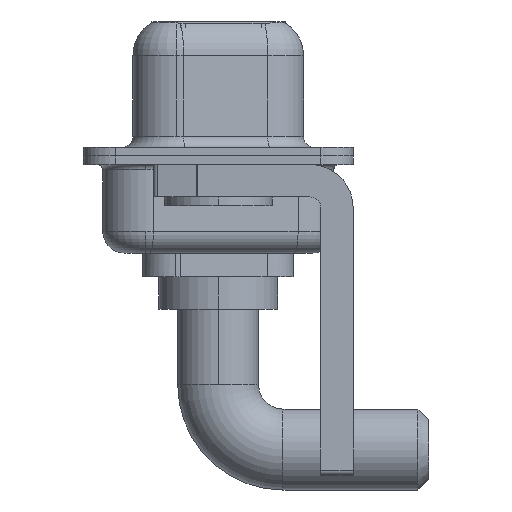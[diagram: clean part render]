
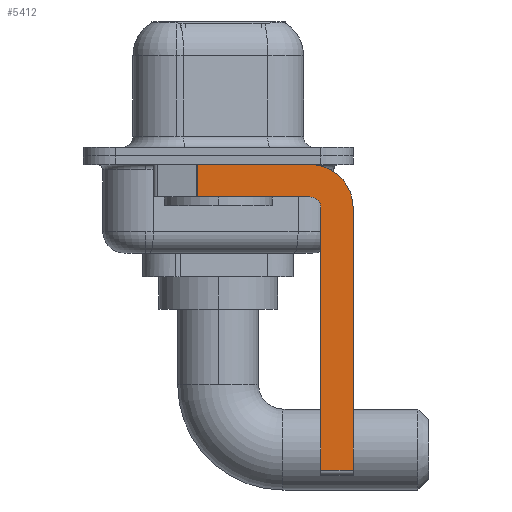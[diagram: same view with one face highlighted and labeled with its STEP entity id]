
A CAD part, left-side view. The second image highlights one B-rep face of the part: STEP entity #5412.
In plain terms, the highlighted planar face has unit normal (-1, 0, 0).
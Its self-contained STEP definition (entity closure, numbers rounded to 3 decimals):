
#215 = VERTEX_POINT ( 'NONE', #4881 ) ;
#233 = DIRECTION ( 'NONE',  ( 0., 0., 1. ) ) ;
#318 = ORIENTED_EDGE ( 'NONE', *, *, #12739, .F. ) ;
#354 = AXIS2_PLACEMENT_3D ( 'NONE', #10210, #6829, #233 ) ;
#401 = VERTEX_POINT ( 'NONE', #9408 ) ;
#510 = EDGE_CURVE ( 'NONE', #3504, #9815, #6223, .T. ) ;
#586 = LINE ( 'NONE', #10084, #4922 ) ;
#731 = VERTEX_POINT ( 'NONE', #3389 ) ;
#924 = VECTOR ( 'NONE', #4280, 1000. ) ;
#963 = VERTEX_POINT ( 'NONE', #9392 ) ;
#1815 = ORIENTED_EDGE ( 'NONE', *, *, #3569, .F. ) ;
#1819 = DIRECTION ( 'NONE',  ( 1., 0., 0. ) ) ;
#1864 = LINE ( 'NONE', #13706, #4674 ) ;
#2394 = VERTEX_POINT ( 'NONE', #5501 ) ;
#2588 = CARTESIAN_POINT ( 'NONE',  ( -2.9, 0.978, -0.4 ) ) ;
#3221 = EDGE_CURVE ( 'NONE', #3504, #401, #6413, .T. ) ;
#3389 = CARTESIAN_POINT ( 'NONE',  ( -2.9, -4.75, -2.4 ) ) ;
#3504 = VERTEX_POINT ( 'NONE', #2588 ) ;
#3560 = VECTOR ( 'NONE', #4054, 1000. ) ;
#3569 = EDGE_CURVE ( 'NONE', #215, #731, #9084, .T. ) ;
#3638 = DIRECTION ( 'NONE',  ( 0., 0., 1. ) ) ;
#4054 = DIRECTION ( 'NONE',  ( 0., 0., -1. ) ) ;
#4280 = DIRECTION ( 'NONE',  ( 0., -1., 0. ) ) ;
#4385 = ORIENTED_EDGE ( 'NONE', *, *, #10401, .T. ) ;
#4420 = VECTOR ( 'NONE', #8425, 1000. ) ;
#4551 = DIRECTION ( 'NONE',  ( 0., 0., -1. ) ) ;
#4674 = VECTOR ( 'NONE', #13566, 1000. ) ;
#4881 = CARTESIAN_POINT ( 'NONE',  ( -2.9, -4.75, -14.55 ) ) ;
#4912 = CARTESIAN_POINT ( 'NONE',  ( -2.9, 0.978, -1.9 ) ) ;
#4917 = DIRECTION ( 'NONE',  ( 0., 1., 0. ) ) ;
#4922 = VECTOR ( 'NONE', #4917, 1000. ) ;
#4967 = ORIENTED_EDGE ( 'NONE', *, *, #3221, .F. ) ;
#4977 = CARTESIAN_POINT ( 'NONE',  ( -2.9, -4.75, -14.8 ) ) ;
#5160 = CARTESIAN_POINT ( 'NONE',  ( -2.9, 0.978, -1.9 ) ) ;
#5412 = ADVANCED_FACE ( 'NONE', ( #12219 ), #8739, .F. ) ;
#5501 = CARTESIAN_POINT ( 'NONE',  ( -2.9, -4.25, -1.9 ) ) ;
#5654 = ORIENTED_EDGE ( 'NONE', *, *, #9717, .F. ) ;
#6118 = CARTESIAN_POINT ( 'NONE',  ( -2.9, -4.25, -2.4 ) ) ;
#6223 = LINE ( 'NONE', #5160, #4420 ) ;
#6413 = LINE ( 'NONE', #8612, #924 ) ;
#6829 = DIRECTION ( 'NONE',  ( -1., 0., 0. ) ) ;
#7475 = ORIENTED_EDGE ( 'NONE', *, *, #13992, .F. ) ;
#7681 = DIRECTION ( 'NONE',  ( 1., 0., 0. ) ) ;
#8119 = DIRECTION ( 'NONE',  ( 0., 0., -1. ) ) ;
#8425 = DIRECTION ( 'NONE',  ( 0., 0., -1. ) ) ;
#8444 = LINE ( 'NONE', #12781, #3560 ) ;
#8612 = CARTESIAN_POINT ( 'NONE',  ( -2.9, 3., -0.4 ) ) ;
#8739 = PLANE ( 'NONE',  #9556 ) ;
#8808 = CARTESIAN_POINT ( 'NONE',  ( -2.9, -4.25, -2.4 ) ) ;
#9084 = LINE ( 'NONE', #4977, #13875 ) ;
#9392 = CARTESIAN_POINT ( 'NONE',  ( -2.9, -6.25, -2.4 ) ) ;
#9408 = CARTESIAN_POINT ( 'NONE',  ( -2.9, -4.25, -0.4 ) ) ;
#9468 = CIRCLE ( 'NONE', #11288, 2. ) ;
#9556 = AXIS2_PLACEMENT_3D ( 'NONE', #8808, #7681, #4551 ) ;
#9717 = EDGE_CURVE ( 'NONE', #731, #2394, #10082, .T. ) ;
#9815 = VERTEX_POINT ( 'NONE', #4912 ) ;
#10082 = CIRCLE ( 'NONE', #354, 0.5 ) ;
#10084 = CARTESIAN_POINT ( 'NONE',  ( -2.9, -4.25, -1.9 ) ) ;
#10210 = CARTESIAN_POINT ( 'NONE',  ( -2.9, -4.25, -2.4 ) ) ;
#10401 = EDGE_CURVE ( 'NONE', #215, #11732, #1864, .T. ) ;
#10906 = ORIENTED_EDGE ( 'NONE', *, *, #510, .T. ) ;
#11154 = EDGE_CURVE ( 'NONE', #2394, #9815, #586, .T. ) ;
#11288 = AXIS2_PLACEMENT_3D ( 'NONE', #6118, #1819, #8119 ) ;
#11355 = EDGE_LOOP ( 'NONE', ( #4967, #10906, #13759, #5654, #1815, #4385, #318, #7475 ) ) ;
#11732 = VERTEX_POINT ( 'NONE', #12633 ) ;
#12219 = FACE_OUTER_BOUND ( 'NONE', #11355, .T. ) ;
#12633 = CARTESIAN_POINT ( 'NONE',  ( -2.9, -6.25, -14.55 ) ) ;
#12739 = EDGE_CURVE ( 'NONE', #963, #11732, #8444, .T. ) ;
#12781 = CARTESIAN_POINT ( 'NONE',  ( -2.9, -6.25, -2.4 ) ) ;
#13566 = DIRECTION ( 'NONE',  ( 0., -1., 0. ) ) ;
#13706 = CARTESIAN_POINT ( 'NONE',  ( -2.9, -4.25, -14.55 ) ) ;
#13759 = ORIENTED_EDGE ( 'NONE', *, *, #11154, .F. ) ;
#13875 = VECTOR ( 'NONE', #3638, 1000. ) ;
#13992 = EDGE_CURVE ( 'NONE', #401, #963, #9468, .T. ) ;
